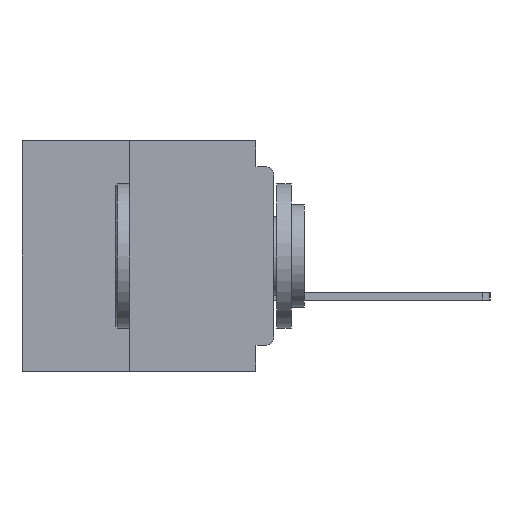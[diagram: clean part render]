
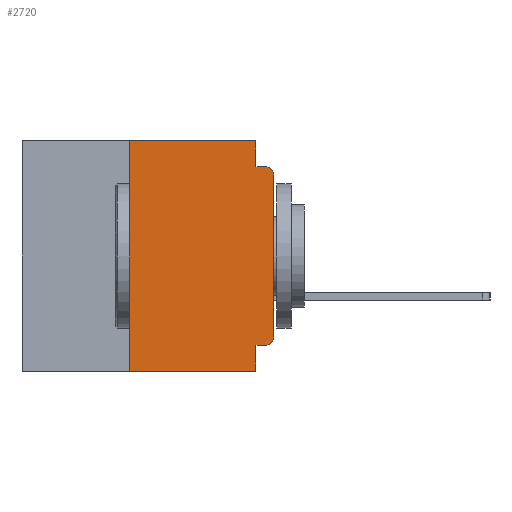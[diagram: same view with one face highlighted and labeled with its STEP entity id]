
A CAD part, left-side view. The second image highlights one B-rep face of the part: STEP entity #2720.
In plain terms, the highlighted planar face has unit normal (-1, 0, 0).
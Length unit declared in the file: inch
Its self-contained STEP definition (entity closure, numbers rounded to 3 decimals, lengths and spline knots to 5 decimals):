
#994 = DIRECTION ( 'NONE',  ( 1., 0., 0. ) ) ;
#1470 = CIRCLE ( 'NONE', #50388, 0.015 ) ;
#1498 = DIRECTION ( 'NONE',  ( 0., 1., 0. ) ) ;
#2720 = ADVANCED_FACE ( 'NONE', ( #34628 ), #49662, .F. ) ;
#2768 = LINE ( 'NONE', #5601, #33967 ) ;
#2803 = CARTESIAN_POINT ( 'NONE',  ( 0., 0., -0.045 ) ) ;
#3635 = EDGE_CURVE ( 'NONE', #42380, #47381, #1470, .T. ) ;
#4238 = VECTOR ( 'NONE', #45938, 39.37008 ) ;
#4594 = CARTESIAN_POINT ( 'NONE',  ( 0., 0.031, 0. ) ) ;
#5589 = CARTESIAN_POINT ( 'NONE',  ( 0., 0.031, 0. ) ) ;
#5601 = CARTESIAN_POINT ( 'NONE',  ( 0., 0., -0.355 ) ) ;
#5698 = VECTOR ( 'NONE', #36991, 39.37008 ) ;
#6383 = VERTEX_POINT ( 'NONE', #18067 ) ;
#9025 = CARTESIAN_POINT ( 'NONE',  ( 0., 0.031, -0.045 ) ) ;
#9222 = EDGE_CURVE ( 'NONE', #6383, #16231, #40436, .T. ) ;
#9305 = EDGE_LOOP ( 'NONE', ( #29524, #29156, #33350, #45571, #44460, #9876, #13652, #26755, #37660, #24984 ) ) ;
#9876 = ORIENTED_EDGE ( 'NONE', *, *, #49566, .F. ) ;
#11096 = CARTESIAN_POINT ( 'NONE',  ( 0., 0.015, -0.34 ) ) ;
#11875 = CARTESIAN_POINT ( 'NONE',  ( 0., 0.437, -0.4 ) ) ;
#12679 = VECTOR ( 'NONE', #31330, 39.37008 ) ;
#13632 = CARTESIAN_POINT ( 'NONE',  ( 0., 0.015, -0.06 ) ) ;
#13652 = ORIENTED_EDGE ( 'NONE', *, *, #37193, .T. ) ;
#15188 = DIRECTION ( 'NONE',  ( 0., 0., -1. ) ) ;
#15243 = DIRECTION ( 'NONE',  ( 0., 0., 1. ) ) ;
#15752 = CARTESIAN_POINT ( 'NONE',  ( 0., 0., -0.06 ) ) ;
#16231 = VERTEX_POINT ( 'NONE', #45376 ) ;
#17234 = EDGE_CURVE ( 'NONE', #23081, #19132, #48368, .T. ) ;
#17751 = DIRECTION ( 'NONE',  ( 0., 0., -1. ) ) ;
#18067 = CARTESIAN_POINT ( 'NONE',  ( 0., 0.031, -0.355 ) ) ;
#18302 = VECTOR ( 'NONE', #40293, 39.37008 ) ;
#18320 = EDGE_CURVE ( 'NONE', #47381, #23081, #48892, .T. ) ;
#18499 = VERTEX_POINT ( 'NONE', #34153 ) ;
#18691 = VERTEX_POINT ( 'NONE', #32239 ) ;
#19132 = VERTEX_POINT ( 'NONE', #38886 ) ;
#19758 = LINE ( 'NONE', #4594, #50796 ) ;
#20800 = EDGE_CURVE ( 'NONE', #51417, #19132, #42547, .T. ) ;
#23081 = VERTEX_POINT ( 'NONE', #15752 ) ;
#24566 = DIRECTION ( 'NONE',  ( 0., 0., -1. ) ) ;
#24984 = ORIENTED_EDGE ( 'NONE', *, *, #3635, .T. ) ;
#25995 = CARTESIAN_POINT ( 'NONE',  ( 0., 0.015, -0.355 ) ) ;
#26755 = ORIENTED_EDGE ( 'NONE', *, *, #9222, .F. ) ;
#28872 = VERTEX_POINT ( 'NONE', #5589 ) ;
#29036 = CARTESIAN_POINT ( 'NONE',  ( 0., 0., 0. ) ) ;
#29156 = ORIENTED_EDGE ( 'NONE', *, *, #17234, .T. ) ;
#29524 = ORIENTED_EDGE ( 'NONE', *, *, #18320, .T. ) ;
#29537 = DIRECTION ( 'NONE',  ( 0., 0., -1. ) ) ;
#31330 = DIRECTION ( 'NONE',  ( 0., -1., 0. ) ) ;
#32239 = CARTESIAN_POINT ( 'NONE',  ( 0., 0.25, -0.4 ) ) ;
#32847 = VECTOR ( 'NONE', #24566, 39.37008 ) ;
#33350 = ORIENTED_EDGE ( 'NONE', *, *, #20800, .F. ) ;
#33442 = CARTESIAN_POINT ( 'NONE',  ( 0., 0.437, 0. ) ) ;
#33502 = LINE ( 'NONE', #35523, #43006 ) ;
#33967 = VECTOR ( 'NONE', #1498, 39.37008 ) ;
#34153 = CARTESIAN_POINT ( 'NONE',  ( 0., 0.25, 0. ) ) ;
#34174 = EDGE_CURVE ( 'NONE', #28872, #51417, #19758, .T. ) ;
#34628 = FACE_OUTER_BOUND ( 'NONE', #9305, .T. ) ;
#35523 = CARTESIAN_POINT ( 'NONE',  ( 0., 0.25, -0.4 ) ) ;
#36681 = LINE ( 'NONE', #41900, #4238 ) ;
#36991 = DIRECTION ( 'NONE',  ( 0., 0., 1. ) ) ;
#37193 = EDGE_CURVE ( 'NONE', #18691, #16231, #39905, .T. ) ;
#37660 = ORIENTED_EDGE ( 'NONE', *, *, #39251, .F. ) ;
#38886 = CARTESIAN_POINT ( 'NONE',  ( 0., 0.015, -0.045 ) ) ;
#39251 = EDGE_CURVE ( 'NONE', #42380, #6383, #2768, .T. ) ;
#39527 = DIRECTION ( 'NONE',  ( -1., 0., 0. ) ) ;
#39905 = LINE ( 'NONE', #11875, #18302 ) ;
#40293 = DIRECTION ( 'NONE',  ( 0., -1., 0. ) ) ;
#40436 = LINE ( 'NONE', #40740, #32847 ) ;
#40740 = CARTESIAN_POINT ( 'NONE',  ( 0., 0.031, -0.4 ) ) ;
#41900 = CARTESIAN_POINT ( 'NONE',  ( 0., 0.437, 0. ) ) ;
#42067 = DIRECTION ( 'NONE',  ( -1., 0., 0. ) ) ;
#42234 = AXIS2_PLACEMENT_3D ( 'NONE', #13632, #42067, #17751 ) ;
#42380 = VERTEX_POINT ( 'NONE', #25995 ) ;
#42547 = LINE ( 'NONE', #2803, #12679 ) ;
#43006 = VECTOR ( 'NONE', #15243, 39.37008 ) ;
#44460 = ORIENTED_EDGE ( 'NONE', *, *, #49311, .F. ) ;
#45248 = DIRECTION ( 'NONE',  ( 0., 0., -1. ) ) ;
#45376 = CARTESIAN_POINT ( 'NONE',  ( 0., 0.031, -0.4 ) ) ;
#45571 = ORIENTED_EDGE ( 'NONE', *, *, #34174, .F. ) ;
#45938 = DIRECTION ( 'NONE',  ( 0., -1., 0. ) ) ;
#47381 = VERTEX_POINT ( 'NONE', #48125 ) ;
#48125 = CARTESIAN_POINT ( 'NONE',  ( 0., 0., -0.34 ) ) ;
#48368 = CIRCLE ( 'NONE', #42234, 0.015 ) ;
#48892 = LINE ( 'NONE', #29036, #5698 ) ;
#49311 = EDGE_CURVE ( 'NONE', #18499, #28872, #36681, .T. ) ;
#49566 = EDGE_CURVE ( 'NONE', #18691, #18499, #33502, .T. ) ;
#49662 = PLANE ( 'NONE',  #50695 ) ;
#50388 = AXIS2_PLACEMENT_3D ( 'NONE', #11096, #39527, #15188 ) ;
#50695 = AXIS2_PLACEMENT_3D ( 'NONE', #33442, #994, #29537 ) ;
#50796 = VECTOR ( 'NONE', #45248, 39.37008 ) ;
#51417 = VERTEX_POINT ( 'NONE', #9025 ) ;
